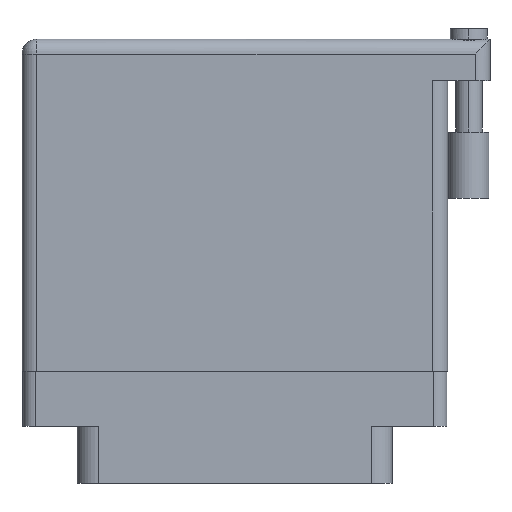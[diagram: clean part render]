
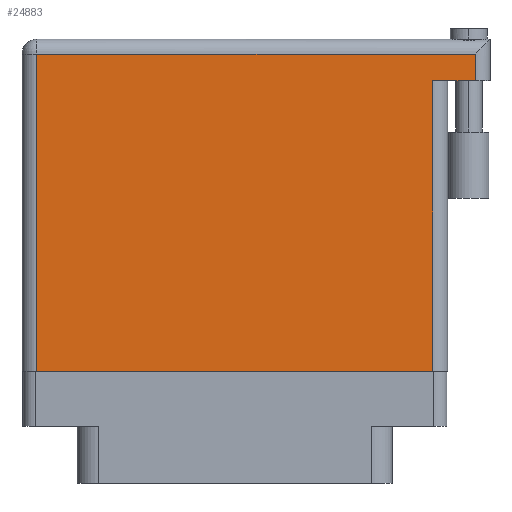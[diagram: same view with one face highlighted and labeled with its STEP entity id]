
A CAD part, front view. The second image highlights one B-rep face of the part: STEP entity #24883.
In plain terms, the highlighted face is planar.
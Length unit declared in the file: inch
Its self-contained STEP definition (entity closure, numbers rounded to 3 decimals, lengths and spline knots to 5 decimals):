
#1906 = CARTESIAN_POINT ( 'NONE',  ( 1.938, 1.369, 0. ) ) ;
#2089 = EDGE_CURVE ( 'NONE', #26615, #2123, #34421, .T. ) ;
#2123 = VERTEX_POINT ( 'NONE', #23208 ) ;
#2161 = DIRECTION ( 'NONE',  ( 0., 1., 0. ) ) ;
#3440 = CARTESIAN_POINT ( 'NONE',  ( 0.07, 1.496, 0. ) ) ;
#4902 = VERTEX_POINT ( 'NONE', #32385 ) ;
#6118 = FACE_OUTER_BOUND ( 'NONE', #29207, .T. ) ;
#6379 = EDGE_CURVE ( 'NONE', #26641, #4902, #14203, .T. ) ;
#6478 = EDGE_CURVE ( 'NONE', #22052, #26615, #22132, .T. ) ;
#7702 = DIRECTION ( 'NONE',  ( 1., 0., 0. ) ) ;
#8153 = CARTESIAN_POINT ( 'NONE',  ( 2.138, 1.566, 0. ) ) ;
#10751 = DIRECTION ( 'NONE',  ( 0., 0., -1. ) ) ;
#11005 = CARTESIAN_POINT ( 'NONE',  ( 0., 1.566, 0. ) ) ;
#11449 = DIRECTION ( 'NONE',  ( 0., 1., 0. ) ) ;
#12344 = VECTOR ( 'NONE', #2161, 39.37008 ) ;
#14001 = DIRECTION ( 'NONE',  ( 0., -1., 0. ) ) ;
#14203 = LINE ( 'NONE', #22978, #26771 ) ;
#15641 = CARTESIAN_POINT ( 'NONE',  ( 0., 1.496, 0. ) ) ;
#16505 = ORIENTED_EDGE ( 'NONE', *, *, #26012, .T. ) ;
#16759 = PLANE ( 'NONE',  #32637 ) ;
#18988 = CARTESIAN_POINT ( 'NONE',  ( 2.138, 1.369, 0. ) ) ;
#20132 = DIRECTION ( 'NONE',  ( -1., 0., 0. ) ) ;
#21635 = DIRECTION ( 'NONE',  ( -1., 0., 0. ) ) ;
#22052 = VERTEX_POINT ( 'NONE', #3440 ) ;
#22132 = LINE ( 'NONE', #25852, #33805 ) ;
#22788 = VECTOR ( 'NONE', #7702, 39.37008 ) ;
#22978 = CARTESIAN_POINT ( 'NONE',  ( 2.208, 1.369, 0. ) ) ;
#22989 = EDGE_CURVE ( 'NONE', #2123, #4902, #32406, .T. ) ;
#23208 = CARTESIAN_POINT ( 'NONE',  ( 1.938, 0., 0. ) ) ;
#24184 = LINE ( 'NONE', #15641, #26547 ) ;
#24883 = ADVANCED_FACE ( 'NONE', ( #6118 ), #16759, .F. ) ;
#25477 = ORIENTED_EDGE ( 'NONE', *, *, #6379, .F. ) ;
#25574 = CARTESIAN_POINT ( 'NONE',  ( 0., 0., 0. ) ) ;
#25852 = CARTESIAN_POINT ( 'NONE',  ( 0.07, 0., 0. ) ) ;
#26012 = EDGE_CURVE ( 'NONE', #36987, #22052, #24184, .T. ) ;
#26547 = VECTOR ( 'NONE', #21635, 39.37008 ) ;
#26615 = VERTEX_POINT ( 'NONE', #36715 ) ;
#26641 = VERTEX_POINT ( 'NONE', #18988 ) ;
#26771 = VECTOR ( 'NONE', #20132, 39.37008 ) ;
#27257 = ORIENTED_EDGE ( 'NONE', *, *, #22989, .T. ) ;
#27632 = ORIENTED_EDGE ( 'NONE', *, *, #2089, .T. ) ;
#29073 = VECTOR ( 'NONE', #11449, 39.37008 ) ;
#29207 = EDGE_LOOP ( 'NONE', ( #27632, #27257, #25477, #32234, #16505, #33366 ) ) ;
#32234 = ORIENTED_EDGE ( 'NONE', *, *, #34159, .T. ) ;
#32385 = CARTESIAN_POINT ( 'NONE',  ( 1.938, 1.369, 0. ) ) ;
#32406 = LINE ( 'NONE', #1906, #12344 ) ;
#32637 = AXIS2_PLACEMENT_3D ( 'NONE', #11005, #10751, #34731 ) ;
#33366 = ORIENTED_EDGE ( 'NONE', *, *, #6478, .T. ) ;
#33805 = VECTOR ( 'NONE', #14001, 39.37008 ) ;
#34159 = EDGE_CURVE ( 'NONE', #26641, #36987, #37030, .T. ) ;
#34421 = LINE ( 'NONE', #25574, #22788 ) ;
#34731 = DIRECTION ( 'NONE',  ( -1., 0., 0. ) ) ;
#36683 = CARTESIAN_POINT ( 'NONE',  ( 2.138, 1.496, 0. ) ) ;
#36715 = CARTESIAN_POINT ( 'NONE',  ( 0.07, 0., 0. ) ) ;
#36987 = VERTEX_POINT ( 'NONE', #36683 ) ;
#37030 = LINE ( 'NONE', #8153, #29073 ) ;
